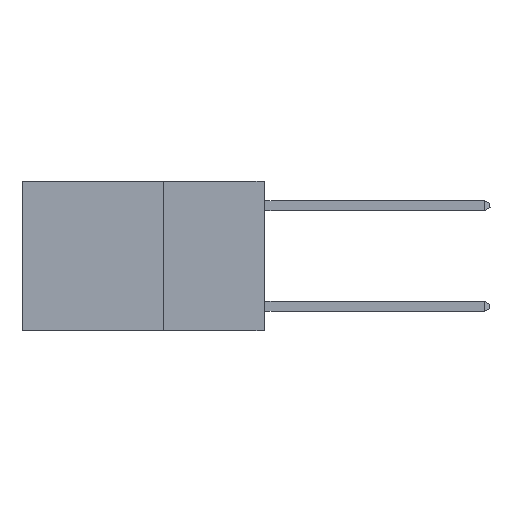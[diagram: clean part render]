
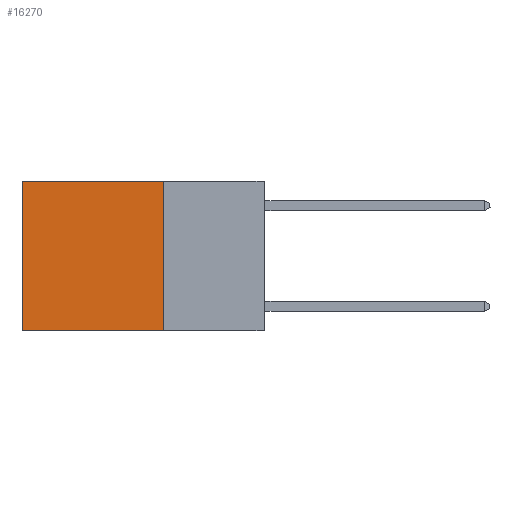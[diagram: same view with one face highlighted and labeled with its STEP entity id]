
A CAD part, left-side view. The second image highlights one B-rep face of the part: STEP entity #16270.
In plain terms, the highlighted planar face has unit normal (-1, 0, 0).
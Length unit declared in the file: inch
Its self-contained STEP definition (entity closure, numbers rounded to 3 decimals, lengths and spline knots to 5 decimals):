
#107 = EDGE_CURVE ( 'NONE', #2393, #20806, #13159, .T. ) ;
#1359 = VECTOR ( 'NONE', #7810, 39.37008 ) ;
#2390 = CARTESIAN_POINT ( 'NONE',  ( 0.2625, 0.6, 0. ) ) ;
#2393 = VERTEX_POINT ( 'NONE', #12133 ) ;
#3350 = DIRECTION ( 'NONE',  ( 0., 1., 0. ) ) ;
#7058 = PLANE ( 'NONE',  #12130 ) ;
#7652 = VECTOR ( 'NONE', #7750, 39.37008 ) ;
#7750 = DIRECTION ( 'NONE',  ( 0., 0., -1. ) ) ;
#7810 = DIRECTION ( 'NONE',  ( 0., 0., -1. ) ) ;
#7812 = VECTOR ( 'NONE', #3350, 39.37008 ) ;
#7931 = ORIENTED_EDGE ( 'NONE', *, *, #21102, .T. ) ;
#8093 = CARTESIAN_POINT ( 'NONE',  ( 0.2625, 0.25, -0.37 ) ) ;
#8602 = VERTEX_POINT ( 'NONE', #2390 ) ;
#9111 = DIRECTION ( 'NONE',  ( 1., 0., 0. ) ) ;
#9268 = ORIENTED_EDGE ( 'NONE', *, *, #23346, .T. ) ;
#9320 = VECTOR ( 'NONE', #10594, 39.37008 ) ;
#10594 = DIRECTION ( 'NONE',  ( 0., 1., 0. ) ) ;
#10685 = EDGE_LOOP ( 'NONE', ( #9268, #14319, #19832, #7931 ) ) ;
#11100 = VERTEX_POINT ( 'NONE', #23044 ) ;
#11153 = DIRECTION ( 'NONE',  ( 0., 0., -1. ) ) ;
#12130 = AXIS2_PLACEMENT_3D ( 'NONE', #17274, #9111, #11153 ) ;
#12133 = CARTESIAN_POINT ( 'NONE',  ( 0.2625, 0.25, -0.37 ) ) ;
#12855 = LINE ( 'NONE', #19991, #1359 ) ;
#13080 = LINE ( 'NONE', #16005, #7652 ) ;
#13159 = LINE ( 'NONE', #8093, #9320 ) ;
#13231 = LINE ( 'NONE', #21620, #7812 ) ;
#14319 = ORIENTED_EDGE ( 'NONE', *, *, #107, .F. ) ;
#14410 = EDGE_CURVE ( 'NONE', #11100, #2393, #13080, .T. ) ;
#16005 = CARTESIAN_POINT ( 'NONE',  ( 0.2625, 0.25, 0. ) ) ;
#16270 = ADVANCED_FACE ( 'NONE', ( #17714 ), #7058, .F. ) ;
#17274 = CARTESIAN_POINT ( 'NONE',  ( 0.2625, 0.25, 0. ) ) ;
#17714 = FACE_OUTER_BOUND ( 'NONE', #10685, .T. ) ;
#19832 = ORIENTED_EDGE ( 'NONE', *, *, #14410, .F. ) ;
#19991 = CARTESIAN_POINT ( 'NONE',  ( 0.2625, 0.6, 0. ) ) ;
#20806 = VERTEX_POINT ( 'NONE', #24680 ) ;
#21102 = EDGE_CURVE ( 'NONE', #11100, #8602, #13231, .T. ) ;
#21620 = CARTESIAN_POINT ( 'NONE',  ( 0.2625, 0.25, 0. ) ) ;
#23044 = CARTESIAN_POINT ( 'NONE',  ( 0.2625, 0.25, 0. ) ) ;
#23346 = EDGE_CURVE ( 'NONE', #8602, #20806, #12855, .T. ) ;
#24680 = CARTESIAN_POINT ( 'NONE',  ( 0.2625, 0.6, -0.37 ) ) ;
